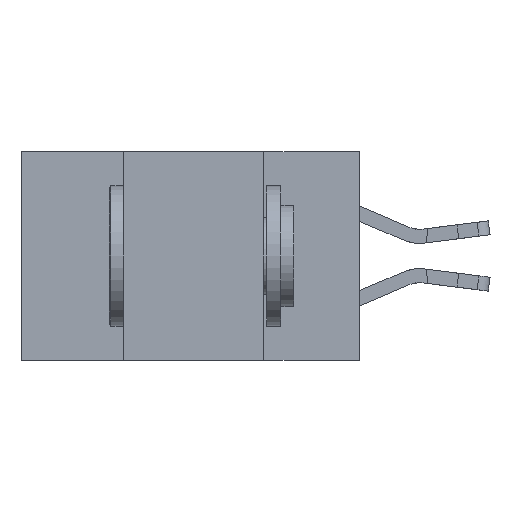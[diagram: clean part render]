
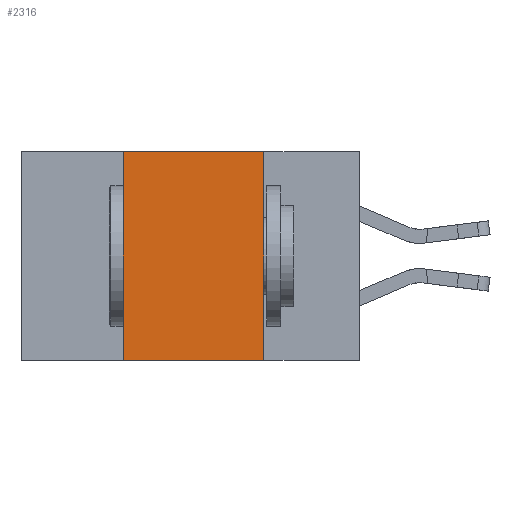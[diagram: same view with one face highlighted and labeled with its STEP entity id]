
A CAD part, left-side view. The second image highlights one B-rep face of the part: STEP entity #2316.
In plain terms, the highlighted planar face has unit normal (-1, 0, 0).
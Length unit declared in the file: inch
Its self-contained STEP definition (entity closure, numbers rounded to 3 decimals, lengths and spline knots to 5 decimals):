
#504 = CARTESIAN_POINT ( 'NONE',  ( 0., 0.42, 0. ) ) ;
#517 = CARTESIAN_POINT ( 'NONE',  ( 0., 0.42, 0. ) ) ;
#1136 = PLANE ( 'NONE',  #8850 ) ;
#1272 = LINE ( 'NONE', #504, #12443 ) ;
#1418 = ORIENTED_EDGE ( 'NONE', *, *, #2866, .T. ) ;
#1995 = CARTESIAN_POINT ( 'NONE',  ( 0., 0.17, 0. ) ) ;
#2316 = ADVANCED_FACE ( 'NONE', ( #6022 ), #1136, .F. ) ;
#2413 = VECTOR ( 'NONE', #11171, 39.37008 ) ;
#2543 = VERTEX_POINT ( 'NONE', #14554 ) ;
#2591 = EDGE_CURVE ( 'NONE', #15060, #13863, #1272, .T. ) ;
#2866 = EDGE_CURVE ( 'NONE', #15060, #5312, #14003, .T. ) ;
#4273 = CARTESIAN_POINT ( 'NONE',  ( 0., 0.6, -0.37 ) ) ;
#4533 = VECTOR ( 'NONE', #7017, 39.37008 ) ;
#4563 = ORIENTED_EDGE ( 'NONE', *, *, #16109, .F. ) ;
#5210 = VECTOR ( 'NONE', #6920, 39.37008 ) ;
#5312 = VERTEX_POINT ( 'NONE', #16613 ) ;
#6022 = FACE_OUTER_BOUND ( 'NONE', #16037, .T. ) ;
#6544 = LINE ( 'NONE', #1995, #5210 ) ;
#6920 = DIRECTION ( 'NONE',  ( 0., 0., -1. ) ) ;
#7017 = DIRECTION ( 'NONE',  ( 0., -1., 0. ) ) ;
#7396 = ORIENTED_EDGE ( 'NONE', *, *, #2591, .F. ) ;
#8850 = AXIS2_PLACEMENT_3D ( 'NONE', #11124, #18347, #14052 ) ;
#8871 = DIRECTION ( 'NONE',  ( 0., 0., 1. ) ) ;
#9516 = ORIENTED_EDGE ( 'NONE', *, *, #17902, .F. ) ;
#9864 = LINE ( 'NONE', #16578, #4533 ) ;
#11124 = CARTESIAN_POINT ( 'NONE',  ( 0., 0.6, 0. ) ) ;
#11171 = DIRECTION ( 'NONE',  ( 0., -1., 0. ) ) ;
#11389 = CARTESIAN_POINT ( 'NONE',  ( 0., 0.42, -0.37 ) ) ;
#12443 = VECTOR ( 'NONE', #8871, 39.37008 ) ;
#13863 = VERTEX_POINT ( 'NONE', #517 ) ;
#14003 = LINE ( 'NONE', #4273, #2413 ) ;
#14052 = DIRECTION ( 'NONE',  ( 0., 0., -1. ) ) ;
#14554 = CARTESIAN_POINT ( 'NONE',  ( 0., 0.17, 0. ) ) ;
#15060 = VERTEX_POINT ( 'NONE', #11389 ) ;
#16037 = EDGE_LOOP ( 'NONE', ( #4563, #9516, #7396, #1418 ) ) ;
#16109 = EDGE_CURVE ( 'NONE', #2543, #5312, #6544, .T. ) ;
#16578 = CARTESIAN_POINT ( 'NONE',  ( 0., 0.6, 0. ) ) ;
#16613 = CARTESIAN_POINT ( 'NONE',  ( 0., 0.17, -0.37 ) ) ;
#17902 = EDGE_CURVE ( 'NONE', #13863, #2543, #9864, .T. ) ;
#18347 = DIRECTION ( 'NONE',  ( 1., 0., 0. ) ) ;
